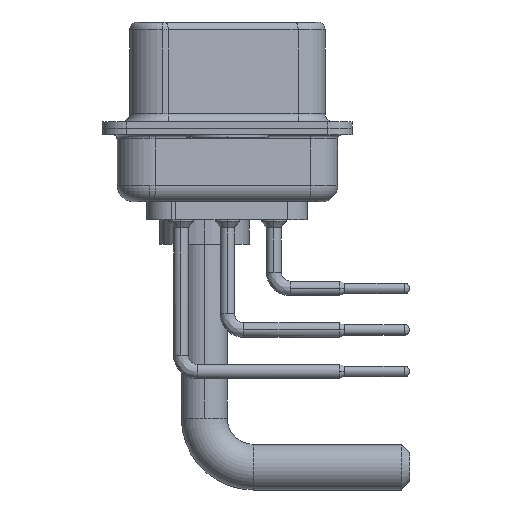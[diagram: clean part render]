
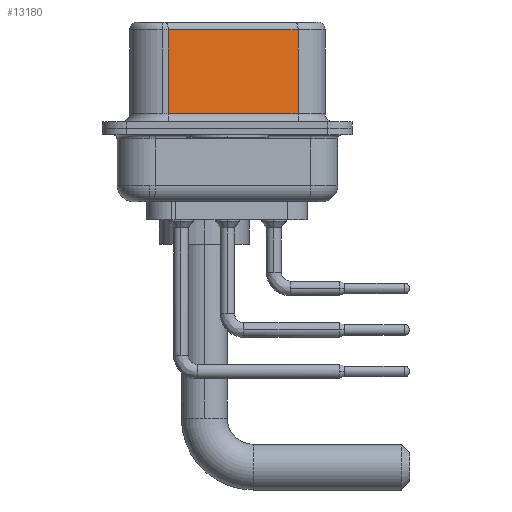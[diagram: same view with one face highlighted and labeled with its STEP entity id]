
A CAD part, left-side view. The second image highlights one B-rep face of the part: STEP entity #13180.
In plain terms, the highlighted planar face has unit normal (-0.985, -0.174, 0).
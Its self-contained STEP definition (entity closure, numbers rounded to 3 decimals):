
#3 = ORIENTED_EDGE ( 'NONE', *, *, #29291, .F. ) ;
#465 = VECTOR ( 'NONE', #30194, 1000. ) ;
#2837 = DIRECTION ( 'NONE',  ( -0.174, 0.985, 0. ) ) ;
#2881 = AXIS2_PLACEMENT_3D ( 'NONE', #5796, #29145, #2837 ) ;
#3012 = CARTESIAN_POINT ( 'NONE',  ( 5.132, -4.322, 0.9 ) ) ;
#3211 = VECTOR ( 'NONE', #31475, 1000. ) ;
#5115 = FACE_OUTER_BOUND ( 'NONE', #9352, .T. ) ;
#5586 = CARTESIAN_POINT ( 'NONE',  ( 5.132, -4.322, 0.9 ) ) ;
#5796 = CARTESIAN_POINT ( 'NONE',  ( 5.132, -4.322, 6.52 ) ) ;
#5869 = VERTEX_POINT ( 'NONE', #5586 ) ;
#7894 = LINE ( 'NONE', #3012, #18429 ) ;
#9274 = EDGE_CURVE ( 'NONE', #21300, #31885, #29376, .T. ) ;
#9310 = CARTESIAN_POINT ( 'NONE',  ( 5.132, -4.322, 6.52 ) ) ;
#9352 = EDGE_LOOP ( 'NONE', ( #3, #19810, #28446, #21521 ) ) ;
#10404 = CARTESIAN_POINT ( 'NONE',  ( 3.73, 3.628, 6.52 ) ) ;
#13143 = EDGE_CURVE ( 'NONE', #31885, #5869, #7894, .T. ) ;
#13180 = ADVANCED_FACE ( 'NONE', ( #5115 ), #29320, .F. ) ;
#13633 = DIRECTION ( 'NONE',  ( 0.174, -0.985, 0. ) ) ;
#13989 = LINE ( 'NONE', #27221, #465 ) ;
#16949 = CARTESIAN_POINT ( 'NONE',  ( 5.132, -4.322, 6.02 ) ) ;
#18429 = VECTOR ( 'NONE', #13633, 1000. ) ;
#19810 = ORIENTED_EDGE ( 'NONE', *, *, #23280, .T. ) ;
#20430 = LINE ( 'NONE', #9310, #26876 ) ;
#21300 = VERTEX_POINT ( 'NONE', #28376 ) ;
#21521 = ORIENTED_EDGE ( 'NONE', *, *, #13143, .T. ) ;
#23186 = VERTEX_POINT ( 'NONE', #16949 ) ;
#23280 = EDGE_CURVE ( 'NONE', #23186, #21300, #13989, .T. ) ;
#26876 = VECTOR ( 'NONE', #30556, 1000. ) ;
#27221 = CARTESIAN_POINT ( 'NONE',  ( 5.132, -4.322, 6.02 ) ) ;
#28376 = CARTESIAN_POINT ( 'NONE',  ( 3.73, 3.628, 6.02 ) ) ;
#28446 = ORIENTED_EDGE ( 'NONE', *, *, #9274, .T. ) ;
#29145 = DIRECTION ( 'NONE',  ( 0.985, 0.174, 0. ) ) ;
#29291 = EDGE_CURVE ( 'NONE', #23186, #5869, #20430, .T. ) ;
#29320 = PLANE ( 'NONE',  #2881 ) ;
#29376 = LINE ( 'NONE', #10404, #3211 ) ;
#30194 = DIRECTION ( 'NONE',  ( -0.174, 0.985, 0. ) ) ;
#30556 = DIRECTION ( 'NONE',  ( 0., 0., -1. ) ) ;
#31475 = DIRECTION ( 'NONE',  ( 0., 0., -1. ) ) ;
#31885 = VERTEX_POINT ( 'NONE', #33419 ) ;
#33419 = CARTESIAN_POINT ( 'NONE',  ( 3.73, 3.628, 0.9 ) ) ;
